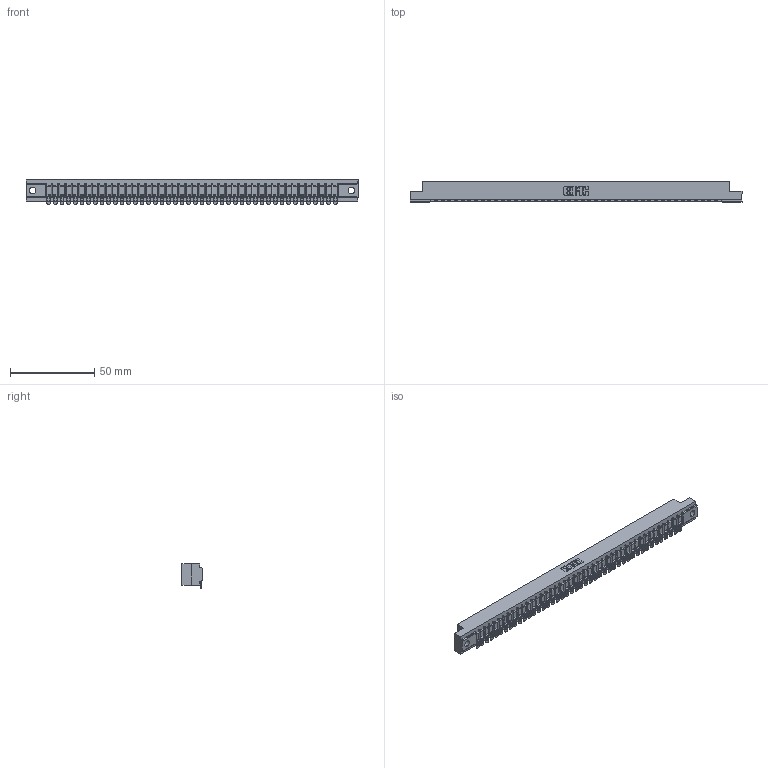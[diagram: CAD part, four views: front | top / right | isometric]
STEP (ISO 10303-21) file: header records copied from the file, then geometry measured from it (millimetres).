
FILE_DESCRIPTION (( 'STEP AP203' ), '1' );
FILE_NAME ('357-044-554-102.STEP', '2019-09-17T11:54:04', ( '' ), ( '' ), 'SwSTEP 2.0', 'SolidWorks 2016', '' );
FILE_SCHEMA (( 'CONFIG_CONTROL_DESIGN' ));
Length unit declared in the file: inch
Products named in the file (3): 357-044-554-102; 307 Part_.128 Dia Mounting Holes; 307-290-002_554
Assembly tree (45 placements, depth 2):
  357-044-554-102
    307 Part_.128 Dia Mounting Holes
    307-290-002_554  x44
Bounding box: 197.36 x 12.01 x 14.52 mm (x, y, z)
Volume: 21062.7 mm3; surface area: 26499.9 mm2
Topology: 45 solids, 45 shells, 3727 faces, 11455 edges, 7514 vertices
Faces by surface type: plane 2094, cylinder 1543, sphere 90
Entity records: 38441 total; most frequent: CARTESIAN_POINT 6486, ORIENTED_EDGE 6476, DIRECTION 6306, EDGE_CURVE 3238, LINE 2474, VECTOR 2474, VERTEX_POINT 2096, AXIS2_PLACEMENT_3D 1916
